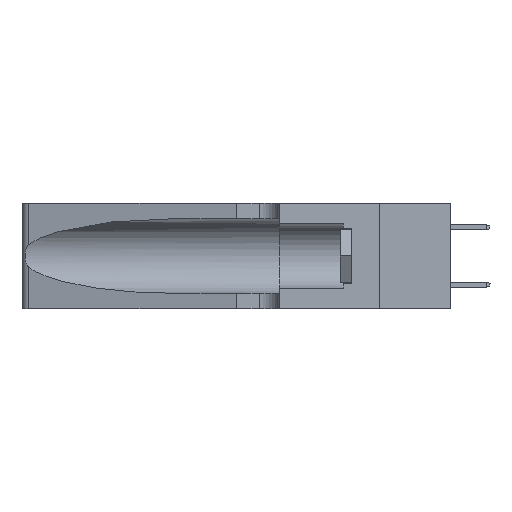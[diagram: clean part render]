
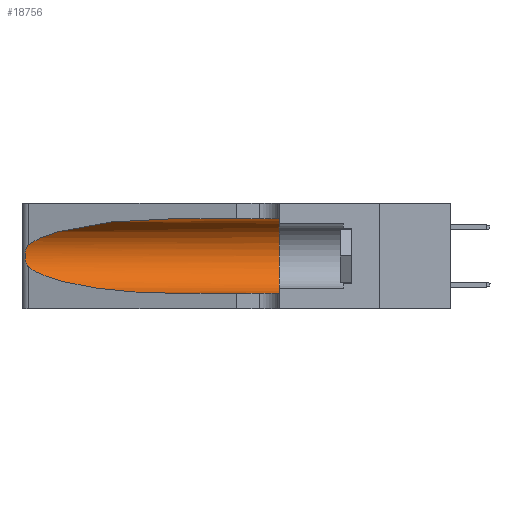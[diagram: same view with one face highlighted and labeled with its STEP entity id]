
A CAD part, left-side view. The second image highlights one B-rep face of the part: STEP entity #18756.
In plain terms, the highlighted cylindrical face has radius 3.308 mm (diameter 6.617 mm), a partial arc.
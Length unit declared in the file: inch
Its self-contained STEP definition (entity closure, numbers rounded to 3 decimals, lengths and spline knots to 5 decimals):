
#501 = CARTESIAN_POINT ( 'NONE',  ( 0.25639, 1.23186, 0.15144 ) ) ;
#881 = CYLINDRICAL_SURFACE ( 'NONE', #18112, 0.13025 ) ;
#1092 =( BOUNDED_CURVE ( )  B_SPLINE_CURVE ( 3, ( #6661, #9557, #12621, #16084 ),
 .UNSPECIFIED., .F., .F. ) 
 B_SPLINE_CURVE_WITH_KNOTS ( ( 4, 4 ),
 ( 1.5708, 2.84003 ),
 .UNSPECIFIED. ) 
 CURVE ( )  GEOMETRIC_REPRESENTATION_ITEM ( )  RATIONAL_B_SPLINE_CURVE ( ( 1., 0.87, 0.87, 1. ) ) 
 REPRESENTATION_ITEM ( '' )  );
#1215 = EDGE_CURVE ( 'NONE', #3542, #15593, #11912, .T. ) ;
#1631 = CARTESIAN_POINT ( 'NONE',  ( 0.25555, 1.22994, 0.2215 ) ) ;
#1836 = CARTESIAN_POINT ( 'NONE',  ( 0.25487, 1.22718, 0.14631 ) ) ;
#2080 = VERTEX_POINT ( 'NONE', #12061 ) ;
#2120 = CARTESIAN_POINT ( 'NONE',  ( 0.2373, 1.15595, 0.08982 ) ) ;
#2400 = CARTESIAN_POINT ( 'NONE',  ( 0.1305, 0.72297, 0.31525 ) ) ;
#2415 = VECTOR ( 'NONE', #8173, 39.37008 ) ;
#3542 = VERTEX_POINT ( 'NONE', #12763 ) ;
#3677 = CARTESIAN_POINT ( 'NONE',  ( 0.25789, 1.23486, 0.15765 ) ) ;
#3951 = ORIENTED_EDGE ( 'NONE', *, *, #15977, .T. ) ;
#5839 = DIRECTION ( 'NONE',  ( 0., 0., 1. ) ) ;
#6149 = CARTESIAN_POINT ( 'NONE',  ( 0.25487, 1.22718, 0.22369 ) ) ;
#6347 = EDGE_LOOP ( 'NONE', ( #16364, #8969, #8702, #3951, #15820, #12747 ) ) ;
#6649 = CARTESIAN_POINT ( 'NONE',  ( 0.18966, 0.96281, 0.05475 ) ) ;
#6661 = CARTESIAN_POINT ( 'NONE',  ( 0.1305, 0.72297, 0.31525 ) ) ;
#6761 = CARTESIAN_POINT ( 'NONE',  ( 0.26017, 1.23833, 0.17102 ) ) ;
#6939 = DIRECTION ( 'NONE',  ( 0., -1., 0. ) ) ;
#7008 = VERTEX_POINT ( 'NONE', #10104 ) ;
#8020 = VERTEX_POINT ( 'NONE', #11285 ) ;
#8173 = DIRECTION ( 'NONE',  ( 0., -1., 0. ) ) ;
#8285 = CARTESIAN_POINT ( 'NONE',  ( 0.25856, 1.23593, 0.16098 ) ) ;
#8702 = ORIENTED_EDGE ( 'NONE', *, *, #12254, .T. ) ;
#8969 = ORIENTED_EDGE ( 'NONE', *, *, #14488, .T. ) ;
#9557 = CARTESIAN_POINT ( 'NONE',  ( 0.18966, 0.96281, 0.31525 ) ) ;
#9651 = CARTESIAN_POINT ( 'NONE',  ( 0.1305, 0.72297, 0.05475 ) ) ;
#10104 = CARTESIAN_POINT ( 'NONE',  ( 0.25487, 1.22718, 0.14631 ) ) ;
#10481 = DIRECTION ( 'NONE',  ( 0., 1., 0. ) ) ;
#11285 = CARTESIAN_POINT ( 'NONE',  ( 0.1305, 0.72297, 0.05475 ) ) ;
#11497 = CARTESIAN_POINT ( 'NONE',  ( 0.25854, 1.2359, 0.20912 ) ) ;
#11601 = LINE ( 'NONE', #14737, #13146 ) ;
#11912 = CIRCLE ( 'NONE', #15152, 0.13025 ) ;
#11991 = DIRECTION ( 'NONE',  ( 0., -1., 0. ) ) ;
#12061 = CARTESIAN_POINT ( 'NONE',  ( 0.25487, 1.22718, 0.22369 ) ) ;
#12254 = EDGE_CURVE ( 'NONE', #7008, #8020, #15762, .T. ) ;
#12609 = CARTESIAN_POINT ( 'NONE',  ( 0.25555, 1.22993, 0.14849 ) ) ;
#12621 = CARTESIAN_POINT ( 'NONE',  ( 0.2373, 1.15595, 0.28018 ) ) ;
#12747 = ORIENTED_EDGE ( 'NONE', *, *, #18751, .F. ) ;
#12763 = CARTESIAN_POINT ( 'NONE',  ( 0.1305, 0.35, 0.31525 ) ) ;
#12804 = CARTESIAN_POINT ( 'NONE',  ( 0.25639, 1.23184, 0.21858 ) ) ;
#12906 = CARTESIAN_POINT ( 'NONE',  ( 0.26075, 1.23896, 0.178 ) ) ;
#13035 = B_SPLINE_CURVE_WITH_KNOTS ( 'NONE', 3,
 ( #6149, #1631, #12804, #17728, #11497, #14137, #19173, #12906, #6761, #8285, #3677, #501, #12609, #17316 ),
 .UNSPECIFIED., .F., .F.,
 ( 4, 2, 2, 2, 2, 2, 4 ),
 ( 0., 0.00027, 0.00053, 0.00107, 0.0016, 0.00187, 0.00214 ),
 .UNSPECIFIED. ) ;
#13146 = VECTOR ( 'NONE', #11991, 39.37008 ) ;
#14137 = CARTESIAN_POINT ( 'NONE',  ( 0.26018, 1.23835, 0.19895 ) ) ;
#14234 = LINE ( 'NONE', #19057, #2415 ) ;
#14488 = EDGE_CURVE ( 'NONE', #2080, #7008, #13035, .T. ) ;
#14737 = CARTESIAN_POINT ( 'NONE',  ( 0.1305, 1.61858, 0.05475 ) ) ;
#14762 = CARTESIAN_POINT ( 'NONE',  ( 0.1305, 0.35, 0.05475 ) ) ;
#15014 = VERTEX_POINT ( 'NONE', #2400 ) ;
#15152 = AXIS2_PLACEMENT_3D ( 'NONE', #19903, #10481, #5839 ) ;
#15593 = VERTEX_POINT ( 'NONE', #14762 ) ;
#15762 =( BOUNDED_CURVE ( )  B_SPLINE_CURVE ( 3, ( #1836, #2120, #6649, #9651 ),
 .UNSPECIFIED., .F., .F. ) 
 B_SPLINE_CURVE_WITH_KNOTS ( ( 4, 4 ),
 ( 3.44316, 4.71239 ),
 .UNSPECIFIED. ) 
 CURVE ( )  GEOMETRIC_REPRESENTATION_ITEM ( )  RATIONAL_B_SPLINE_CURVE ( ( 1., 0.87, 0.87, 1. ) ) 
 REPRESENTATION_ITEM ( '' )  );
#15820 = ORIENTED_EDGE ( 'NONE', *, *, #1215, .F. ) ;
#15977 = EDGE_CURVE ( 'NONE', #8020, #15593, #11601, .T. ) ;
#16084 = CARTESIAN_POINT ( 'NONE',  ( 0.25487, 1.22718, 0.22369 ) ) ;
#16277 = CARTESIAN_POINT ( 'NONE',  ( 0.1305, 1.61858, 0.185 ) ) ;
#16364 = ORIENTED_EDGE ( 'NONE', *, *, #19606, .T. ) ;
#17316 = CARTESIAN_POINT ( 'NONE',  ( 0.25487, 1.22718, 0.14631 ) ) ;
#17615 = FACE_OUTER_BOUND ( 'NONE', #6347, .T. ) ;
#17728 = CARTESIAN_POINT ( 'NONE',  ( 0.25787, 1.23484, 0.2124 ) ) ;
#17925 = DIRECTION ( 'NONE',  ( 0., 0., -1. ) ) ;
#18112 = AXIS2_PLACEMENT_3D ( 'NONE', #16277, #6939, #17925 ) ;
#18751 = EDGE_CURVE ( 'NONE', #15014, #3542, #14234, .T. ) ;
#18756 = ADVANCED_FACE ( 'NONE', ( #17615 ), #881, .F. ) ;
#19057 = CARTESIAN_POINT ( 'NONE',  ( 0.1305, 1.61858, 0.31525 ) ) ;
#19173 = CARTESIAN_POINT ( 'NONE',  ( 0.26075, 1.23896, 0.19203 ) ) ;
#19606 = EDGE_CURVE ( 'NONE', #15014, #2080, #1092, .T. ) ;
#19903 = CARTESIAN_POINT ( 'NONE',  ( 0.1305, 0.35, 0.185 ) ) ;
